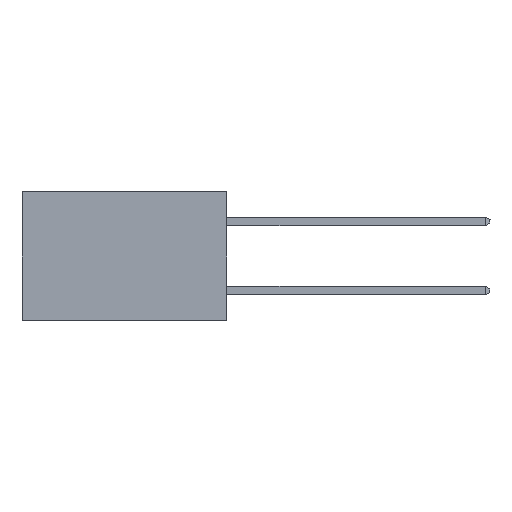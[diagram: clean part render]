
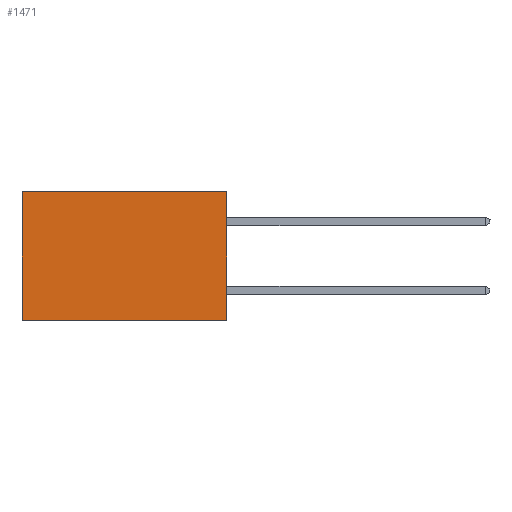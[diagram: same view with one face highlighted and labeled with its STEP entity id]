
A CAD part, left-side view. The second image highlights one B-rep face of the part: STEP entity #1471.
In plain terms, the highlighted planar face has unit normal (-1, 0, 0).
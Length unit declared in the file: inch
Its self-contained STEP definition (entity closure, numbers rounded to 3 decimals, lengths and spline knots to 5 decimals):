
#136 = LINE ( 'NONE', #13383, #8364 ) ;
#896 = CARTESIAN_POINT ( 'NONE',  ( 0.277, 0., -0.37 ) ) ;
#1351 = CARTESIAN_POINT ( 'NONE',  ( 0.277, 0.59, -0.37 ) ) ;
#1471 = ADVANCED_FACE ( 'NONE', ( #9207 ), #18297, .F. ) ;
#1695 = VECTOR ( 'NONE', #8498, 39.37008 ) ;
#2049 = DIRECTION ( 'NONE',  ( 0., 0., -1. ) ) ;
#2214 = LINE ( 'NONE', #20189, #1695 ) ;
#2586 = EDGE_CURVE ( 'NONE', #16140, #11537, #10434, .T. ) ;
#3522 = EDGE_CURVE ( 'NONE', #14541, #11537, #2214, .T. ) ;
#3815 = VERTEX_POINT ( 'NONE', #7513 ) ;
#5921 = EDGE_CURVE ( 'NONE', #3815, #14541, #19780, .T. ) ;
#6112 = ORIENTED_EDGE ( 'NONE', *, *, #14180, .F. ) ;
#6793 = ORIENTED_EDGE ( 'NONE', *, *, #3522, .T. ) ;
#7513 = CARTESIAN_POINT ( 'NONE',  ( 0.277, 0., 0. ) ) ;
#7785 = DIRECTION ( 'NONE',  ( 0., 0., -1. ) ) ;
#8364 = VECTOR ( 'NONE', #2049, 39.37008 ) ;
#8469 = DIRECTION ( 'NONE',  ( 0., 1., 0. ) ) ;
#8498 = DIRECTION ( 'NONE',  ( 0., 0., -1. ) ) ;
#9207 = FACE_OUTER_BOUND ( 'NONE', #20500, .T. ) ;
#10434 = LINE ( 'NONE', #896, #14124 ) ;
#10799 = AXIS2_PLACEMENT_3D ( 'NONE', #14080, #14540, #7785 ) ;
#11537 = VERTEX_POINT ( 'NONE', #1351 ) ;
#11765 = CARTESIAN_POINT ( 'NONE',  ( 0.277, 0., 0. ) ) ;
#13144 = ORIENTED_EDGE ( 'NONE', *, *, #5921, .T. ) ;
#13383 = CARTESIAN_POINT ( 'NONE',  ( 0.277, 0., -0.37 ) ) ;
#14080 = CARTESIAN_POINT ( 'NONE',  ( 0.277, 0., -0.37 ) ) ;
#14124 = VECTOR ( 'NONE', #20660, 39.37008 ) ;
#14180 = EDGE_CURVE ( 'NONE', #3815, #16140, #136, .T. ) ;
#14540 = DIRECTION ( 'NONE',  ( 1., 0., 0. ) ) ;
#14541 = VERTEX_POINT ( 'NONE', #20434 ) ;
#16071 = VECTOR ( 'NONE', #8469, 39.37008 ) ;
#16140 = VERTEX_POINT ( 'NONE', #19387 ) ;
#16293 = ORIENTED_EDGE ( 'NONE', *, *, #2586, .F. ) ;
#18297 = PLANE ( 'NONE',  #10799 ) ;
#19387 = CARTESIAN_POINT ( 'NONE',  ( 0.277, 0., -0.37 ) ) ;
#19780 = LINE ( 'NONE', #11765, #16071 ) ;
#20189 = CARTESIAN_POINT ( 'NONE',  ( 0.277, 0.59, -0.37 ) ) ;
#20434 = CARTESIAN_POINT ( 'NONE',  ( 0.277, 0.59, 0. ) ) ;
#20500 = EDGE_LOOP ( 'NONE', ( #6793, #16293, #6112, #13144 ) ) ;
#20660 = DIRECTION ( 'NONE',  ( 0., 1., 0. ) ) ;
